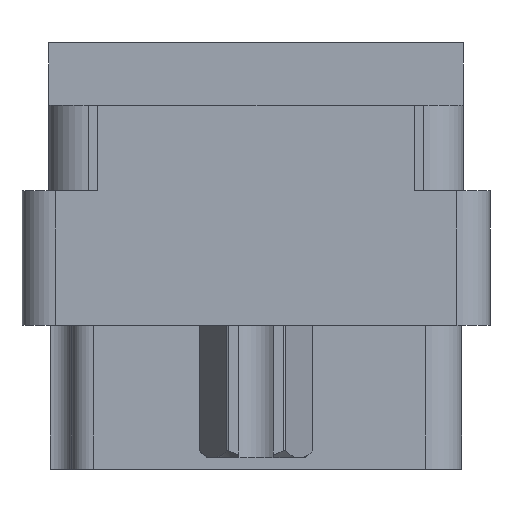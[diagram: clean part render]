
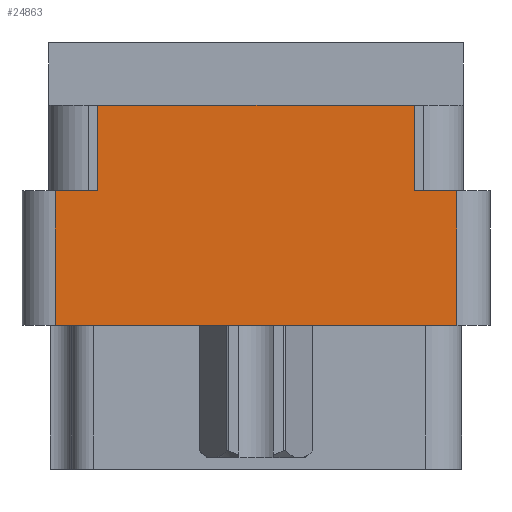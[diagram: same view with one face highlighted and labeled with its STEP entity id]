
A CAD part, left-side view. The second image highlights one B-rep face of the part: STEP entity #24863.
In plain terms, the highlighted planar face has unit normal (-1, 0, 0).
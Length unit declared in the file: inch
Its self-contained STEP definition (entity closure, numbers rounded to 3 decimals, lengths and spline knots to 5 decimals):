
#382 = EDGE_CURVE ( 'NONE', #31709, #42233, #33795, .T. ) ;
#804 = PLANE ( 'NONE',  #35506 ) ;
#1880 = EDGE_CURVE ( 'NONE', #29434, #42233, #12609, .T. ) ;
#2619 = EDGE_CURVE ( 'NONE', #31709, #19222, #5161, .T. ) ;
#3033 = CARTESIAN_POINT ( 'NONE',  ( -1., -0.376, -0.529 ) ) ;
#3425 = VERTEX_POINT ( 'NONE', #37191 ) ;
#3725 = VECTOR ( 'NONE', #37086, 39.37008 ) ;
#4450 = VECTOR ( 'NONE', #18566, 39.37008 ) ;
#4630 = ORIENTED_EDGE ( 'NONE', *, *, #39691, .F. ) ;
#4930 = CARTESIAN_POINT ( 'NONE',  ( -1., 0.438, -0.117 ) ) ;
#5130 = DIRECTION ( 'NONE',  ( 0., -1., 0. ) ) ;
#5161 = LINE ( 'NONE', #22093, #29431 ) ;
#6549 = FACE_OUTER_BOUND ( 'NONE', #34442, .T. ) ;
#8308 = DIRECTION ( 'NONE',  ( 0., 1., 0. ) ) ;
#8347 = DIRECTION ( 'NONE',  ( 0., -1., 0. ) ) ;
#9519 = VERTEX_POINT ( 'NONE', #27085 ) ;
#10040 = CARTESIAN_POINT ( 'NONE',  ( -1., 0., -0.277 ) ) ;
#11856 = VECTOR ( 'NONE', #8347, 39.37008 ) ;
#12609 = LINE ( 'NONE', #21570, #32639 ) ;
#14336 = CARTESIAN_POINT ( 'NONE',  ( -1., -0.438, -0.798 ) ) ;
#15637 = EDGE_CURVE ( 'NONE', #3425, #19671, #41917, .T. ) ;
#16114 = CARTESIAN_POINT ( 'NONE',  ( -1., 0.376, -0.277 ) ) ;
#17123 = DIRECTION ( 'NONE',  ( 0., -1., 0. ) ) ;
#17406 = EDGE_CURVE ( 'NONE', #3425, #39466, #30307, .T. ) ;
#17570 = EDGE_CURVE ( 'NONE', #29434, #19671, #38709, .T. ) ;
#17725 = DIRECTION ( 'NONE',  ( -1., 0., 0. ) ) ;
#18565 = ORIENTED_EDGE ( 'NONE', *, *, #17570, .T. ) ;
#18566 = DIRECTION ( 'NONE',  ( 0., 0., 1. ) ) ;
#19080 = CARTESIAN_POINT ( 'NONE',  ( -1., -0.376, -0.277 ) ) ;
#19222 = VERTEX_POINT ( 'NONE', #31235 ) ;
#19671 = VERTEX_POINT ( 'NONE', #19080 ) ;
#19773 = LINE ( 'NONE', #4930, #11856 ) ;
#20475 = VECTOR ( 'NONE', #43685, 39.37008 ) ;
#21570 = CARTESIAN_POINT ( 'NONE',  ( -1., 0., -0.529 ) ) ;
#22093 = CARTESIAN_POINT ( 'NONE',  ( -1., 0., -0.277 ) ) ;
#23959 = VECTOR ( 'NONE', #36277, 39.37008 ) ;
#24095 = DIRECTION ( 'NONE',  ( 0., 0., 1. ) ) ;
#24863 = ADVANCED_FACE ( 'NONE', ( #6549 ), #804, .T. ) ;
#27085 = CARTESIAN_POINT ( 'NONE',  ( -1., 0.296, -0.117 ) ) ;
#27873 = LINE ( 'NONE', #36801, #20475 ) ;
#27983 = ORIENTED_EDGE ( 'NONE', *, *, #2619, .F. ) ;
#29431 = VECTOR ( 'NONE', #5130, 39.37008 ) ;
#29434 = VERTEX_POINT ( 'NONE', #3033 ) ;
#30173 = CARTESIAN_POINT ( 'NONE',  ( -1., 0.376, -0.798 ) ) ;
#30307 = LINE ( 'NONE', #35118, #4450 ) ;
#31235 = CARTESIAN_POINT ( 'NONE',  ( -1., 0.296, -0.277 ) ) ;
#31373 = ORIENTED_EDGE ( 'NONE', *, *, #382, .T. ) ;
#31709 = VERTEX_POINT ( 'NONE', #16114 ) ;
#32473 = CARTESIAN_POINT ( 'NONE',  ( -1., 0.376, -0.529 ) ) ;
#32639 = VECTOR ( 'NONE', #8308, 39.37008 ) ;
#32900 = CARTESIAN_POINT ( 'NONE',  ( -1., -0.376, -0.798 ) ) ;
#33795 = LINE ( 'NONE', #30173, #3725 ) ;
#34442 = EDGE_LOOP ( 'NONE', ( #27983, #31373, #35651, #18565, #40936, #36170, #4630, #40029 ) ) ;
#35118 = CARTESIAN_POINT ( 'NONE',  ( -1., -0.296, -0.277 ) ) ;
#35506 = AXIS2_PLACEMENT_3D ( 'NONE', #14336, #17725, #24095 ) ;
#35651 = ORIENTED_EDGE ( 'NONE', *, *, #1880, .F. ) ;
#36078 = CARTESIAN_POINT ( 'NONE',  ( -1., -0.296, -0.117 ) ) ;
#36170 = ORIENTED_EDGE ( 'NONE', *, *, #17406, .T. ) ;
#36277 = DIRECTION ( 'NONE',  ( 0., 0., 1. ) ) ;
#36801 = CARTESIAN_POINT ( 'NONE',  ( -1., 0.296, -0.277 ) ) ;
#37086 = DIRECTION ( 'NONE',  ( 0., 0., -1. ) ) ;
#37191 = CARTESIAN_POINT ( 'NONE',  ( -1., -0.296, -0.277 ) ) ;
#37694 = EDGE_CURVE ( 'NONE', #19222, #9519, #27873, .T. ) ;
#38709 = LINE ( 'NONE', #32900, #23959 ) ;
#39466 = VERTEX_POINT ( 'NONE', #36078 ) ;
#39691 = EDGE_CURVE ( 'NONE', #9519, #39466, #19773, .T. ) ;
#40029 = ORIENTED_EDGE ( 'NONE', *, *, #37694, .F. ) ;
#40936 = ORIENTED_EDGE ( 'NONE', *, *, #15637, .F. ) ;
#41917 = LINE ( 'NONE', #10040, #42982 ) ;
#42233 = VERTEX_POINT ( 'NONE', #32473 ) ;
#42982 = VECTOR ( 'NONE', #17123, 39.37008 ) ;
#43685 = DIRECTION ( 'NONE',  ( 0., 0., 1. ) ) ;
